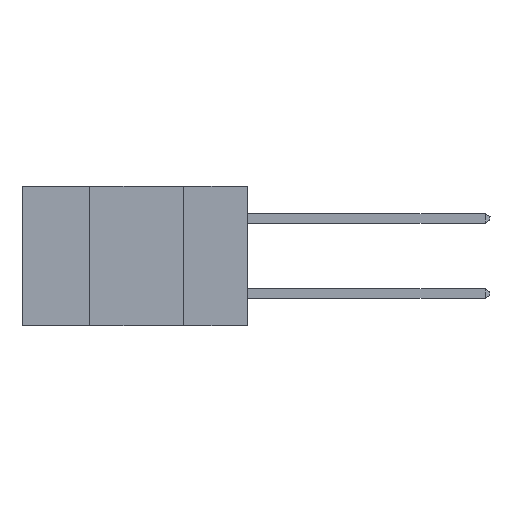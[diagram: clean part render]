
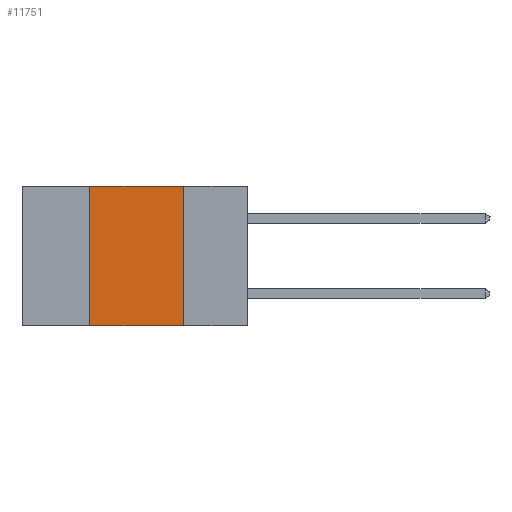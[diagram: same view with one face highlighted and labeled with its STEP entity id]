
A CAD part, left-side view. The second image highlights one B-rep face of the part: STEP entity #11751.
In plain terms, the highlighted planar face has unit normal (-1, 0, 0).
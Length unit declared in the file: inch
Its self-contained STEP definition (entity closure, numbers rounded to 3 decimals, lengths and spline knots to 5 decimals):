
#149 = VERTEX_POINT ( 'NONE', #10105 ) ;
#176 = PLANE ( 'NONE',  #2457 ) ;
#553 = DIRECTION ( 'NONE',  ( 0., 0., -1. ) ) ;
#622 = DIRECTION ( 'NONE',  ( 1., 0., 0. ) ) ;
#1710 = DIRECTION ( 'NONE',  ( 0., 0., -1. ) ) ;
#1713 = ORIENTED_EDGE ( 'NONE', *, *, #11299, .F. ) ;
#2181 = DIRECTION ( 'NONE',  ( 0., -1., 0. ) ) ;
#2457 = AXIS2_PLACEMENT_3D ( 'NONE', #4803, #622, #553 ) ;
#3362 = VECTOR ( 'NONE', #2181, 39.37008 ) ;
#3585 = EDGE_CURVE ( 'NONE', #11879, #9522, #5692, .T. ) ;
#3988 = CARTESIAN_POINT ( 'NONE',  ( 0., 0.42, -0.37 ) ) ;
#4010 = ORIENTED_EDGE ( 'NONE', *, *, #3585, .F. ) ;
#4700 = CARTESIAN_POINT ( 'NONE',  ( 0., 0.17, -0.37 ) ) ;
#4803 = CARTESIAN_POINT ( 'NONE',  ( 0., 0.6, 0. ) ) ;
#5145 = LINE ( 'NONE', #8814, #3362 ) ;
#5692 = LINE ( 'NONE', #14839, #6839 ) ;
#5763 = CARTESIAN_POINT ( 'NONE',  ( 0., 0.42, 0. ) ) ;
#6256 = ORIENTED_EDGE ( 'NONE', *, *, #10964, .F. ) ;
#6458 = EDGE_LOOP ( 'NONE', ( #6256, #4010, #1713, #10634 ) ) ;
#6459 = CARTESIAN_POINT ( 'NONE',  ( 0., 0.17, 0. ) ) ;
#6626 = CARTESIAN_POINT ( 'NONE',  ( 0., 0.17, -0.37 ) ) ;
#6839 = VECTOR ( 'NONE', #9120, 39.37008 ) ;
#6996 = VERTEX_POINT ( 'NONE', #4700 ) ;
#8544 = EDGE_CURVE ( 'NONE', #149, #6996, #5145, .T. ) ;
#8549 = DIRECTION ( 'NONE',  ( 0., 0., 1. ) ) ;
#8814 = CARTESIAN_POINT ( 'NONE',  ( 0., 0.6, -0.37 ) ) ;
#9120 = DIRECTION ( 'NONE',  ( 0., -1., 0. ) ) ;
#9522 = VERTEX_POINT ( 'NONE', #6459 ) ;
#10105 = CARTESIAN_POINT ( 'NONE',  ( 0., 0.42, -0.37 ) ) ;
#10491 = FACE_OUTER_BOUND ( 'NONE', #6458, .T. ) ;
#10634 = ORIENTED_EDGE ( 'NONE', *, *, #8544, .T. ) ;
#10950 = LINE ( 'NONE', #3988, #14183 ) ;
#10964 = EDGE_CURVE ( 'NONE', #9522, #6996, #12327, .T. ) ;
#11299 = EDGE_CURVE ( 'NONE', #149, #11879, #10950, .T. ) ;
#11751 = ADVANCED_FACE ( 'NONE', ( #10491 ), #176, .F. ) ;
#11879 = VERTEX_POINT ( 'NONE', #5763 ) ;
#12327 = LINE ( 'NONE', #6626, #13931 ) ;
#13931 = VECTOR ( 'NONE', #1710, 39.37008 ) ;
#14183 = VECTOR ( 'NONE', #8549, 39.37008 ) ;
#14839 = CARTESIAN_POINT ( 'NONE',  ( 0., 0.6, 0. ) ) ;
